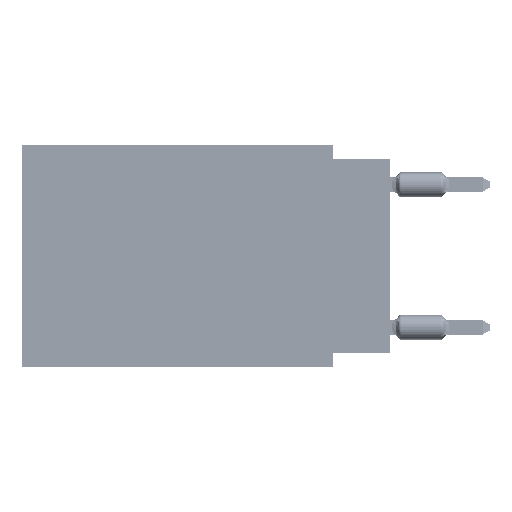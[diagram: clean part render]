
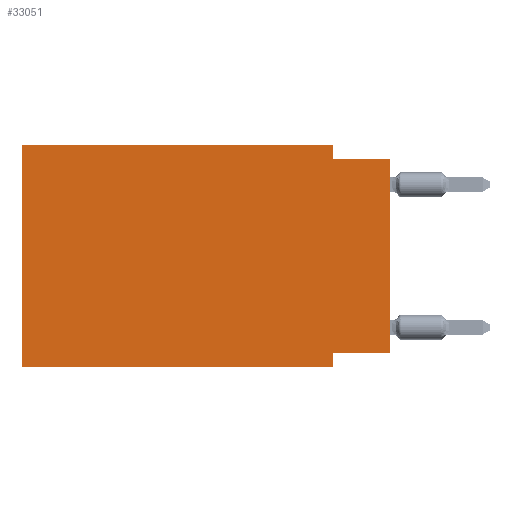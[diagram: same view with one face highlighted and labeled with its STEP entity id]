
A CAD part, left-side view. The second image highlights one B-rep face of the part: STEP entity #33051.
In plain terms, the highlighted planar face has unit normal (-1, 0, 0).
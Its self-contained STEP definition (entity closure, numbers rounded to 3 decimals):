
#873 = CARTESIAN_POINT ( 'NONE',  ( 0., 16.383, 0. ) ) ;
#1755 = VERTEX_POINT ( 'NONE', #80911 ) ;
#2110 = EDGE_CURVE ( 'NONE', #83884, #30209, #72655, .T. ) ;
#7801 = CARTESIAN_POINT ( 'NONE',  ( 0., 16.383, 0. ) ) ;
#10353 = LINE ( 'NONE', #70918, #32037 ) ;
#11198 = CARTESIAN_POINT ( 'NONE',  ( 0., 0., 0. ) ) ;
#11540 = CARTESIAN_POINT ( 'NONE',  ( 0., 2.54, -9.906 ) ) ;
#12314 = ORIENTED_EDGE ( 'NONE', *, *, #60166, .F. ) ;
#12591 = ORIENTED_EDGE ( 'NONE', *, *, #87006, .F. ) ;
#12989 = VECTOR ( 'NONE', #28167, 1000. ) ;
#16115 = LINE ( 'NONE', #64992, #87766 ) ;
#18404 = PLANE ( 'NONE',  #35913 ) ;
#19910 = CARTESIAN_POINT ( 'NONE',  ( 0., 0., -0.635 ) ) ;
#21393 = VECTOR ( 'NONE', #25975, 1000. ) ;
#21594 = EDGE_CURVE ( 'NONE', #63726, #67853, #56403, .T. ) ;
#21846 = CARTESIAN_POINT ( 'NONE',  ( 0., 0., -9.271 ) ) ;
#24048 = LINE ( 'NONE', #85064, #24324 ) ;
#24324 = VECTOR ( 'NONE', #50980, 1000. ) ;
#24879 = EDGE_CURVE ( 'NONE', #83283, #50228, #10353, .T. ) ;
#25975 = DIRECTION ( 'NONE',  ( 0., 0., 1. ) ) ;
#26009 = DIRECTION ( 'NONE',  ( 1., 0., 0. ) ) ;
#27300 = ORIENTED_EDGE ( 'NONE', *, *, #24879, .T. ) ;
#28167 = DIRECTION ( 'NONE',  ( 0., -1., 0. ) ) ;
#30209 = VERTEX_POINT ( 'NONE', #19910 ) ;
#32037 = VECTOR ( 'NONE', #37738, 1000. ) ;
#33051 = ADVANCED_FACE ( 'NONE', ( #39063 ), #18404, .F. ) ;
#33146 = CARTESIAN_POINT ( 'NONE',  ( 0., 2.54, -0.635 ) ) ;
#34312 = ORIENTED_EDGE ( 'NONE', *, *, #39847, .F. ) ;
#35913 = AXIS2_PLACEMENT_3D ( 'NONE', #53825, #26009, #73125 ) ;
#37738 = DIRECTION ( 'NONE',  ( 0., -1., 0. ) ) ;
#37773 = VECTOR ( 'NONE', #69237, 1000. ) ;
#39063 = FACE_OUTER_BOUND ( 'NONE', #53913, .T. ) ;
#39847 = EDGE_CURVE ( 'NONE', #1755, #50228, #65395, .T. ) ;
#42937 = CARTESIAN_POINT ( 'NONE',  ( 0., 16.383, 0. ) ) ;
#43499 = DIRECTION ( 'NONE',  ( 0., 0., -1. ) ) ;
#44649 = EDGE_CURVE ( 'NONE', #83884, #1755, #82540, .T. ) ;
#46849 = VERTEX_POINT ( 'NONE', #33146 ) ;
#50228 = VERTEX_POINT ( 'NONE', #83608 ) ;
#50980 = DIRECTION ( 'NONE',  ( 0., -1., 0. ) ) ;
#53825 = CARTESIAN_POINT ( 'NONE',  ( 0., 16.383, 0. ) ) ;
#53913 = EDGE_LOOP ( 'NONE', ( #54891, #61899, #12591, #82457, #12314, #27300, #34312, #84373 ) ) ;
#54891 = ORIENTED_EDGE ( 'NONE', *, *, #2110, .T. ) ;
#56403 = LINE ( 'NONE', #42937, #12989 ) ;
#58649 = DIRECTION ( 'NONE',  ( 0., 0., -1. ) ) ;
#60166 = EDGE_CURVE ( 'NONE', #83283, #63726, #82698, .T. ) ;
#61899 = ORIENTED_EDGE ( 'NONE', *, *, #83922, .F. ) ;
#63726 = VERTEX_POINT ( 'NONE', #873 ) ;
#64992 = CARTESIAN_POINT ( 'NONE',  ( 0., 2.54, 0. ) ) ;
#65395 = LINE ( 'NONE', #11540, #83450 ) ;
#65685 = CARTESIAN_POINT ( 'NONE',  ( 0., 2.54, 0. ) ) ;
#67853 = VERTEX_POINT ( 'NONE', #65685 ) ;
#69237 = DIRECTION ( 'NONE',  ( 0., 0., 1. ) ) ;
#70918 = CARTESIAN_POINT ( 'NONE',  ( 0., 16.383, -9.906 ) ) ;
#72655 = LINE ( 'NONE', #11198, #21393 ) ;
#73125 = DIRECTION ( 'NONE',  ( 0., 0., -1. ) ) ;
#75373 = DIRECTION ( 'NONE',  ( 0., 1., 0. ) ) ;
#80731 = CARTESIAN_POINT ( 'NONE',  ( 0., 16.383, -9.906 ) ) ;
#80911 = CARTESIAN_POINT ( 'NONE',  ( 0., 2.54, -9.271 ) ) ;
#82094 = CARTESIAN_POINT ( 'NONE',  ( 0., 0., -9.271 ) ) ;
#82457 = ORIENTED_EDGE ( 'NONE', *, *, #21594, .F. ) ;
#82540 = LINE ( 'NONE', #82094, #86665 ) ;
#82698 = LINE ( 'NONE', #7801, #37773 ) ;
#83283 = VERTEX_POINT ( 'NONE', #80731 ) ;
#83450 = VECTOR ( 'NONE', #58649, 1000. ) ;
#83608 = CARTESIAN_POINT ( 'NONE',  ( 0., 2.54, -9.906 ) ) ;
#83884 = VERTEX_POINT ( 'NONE', #21846 ) ;
#83922 = EDGE_CURVE ( 'NONE', #46849, #30209, #24048, .T. ) ;
#84373 = ORIENTED_EDGE ( 'NONE', *, *, #44649, .F. ) ;
#85064 = CARTESIAN_POINT ( 'NONE',  ( 0., 0., -0.635 ) ) ;
#86665 = VECTOR ( 'NONE', #75373, 1000. ) ;
#87006 = EDGE_CURVE ( 'NONE', #67853, #46849, #16115, .T. ) ;
#87766 = VECTOR ( 'NONE', #43499, 1000. ) ;
